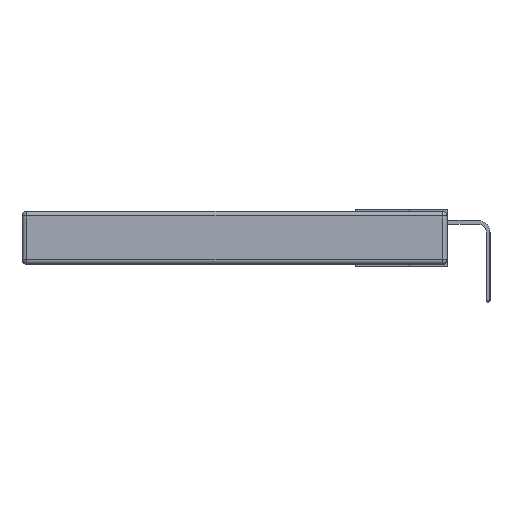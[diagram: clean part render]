
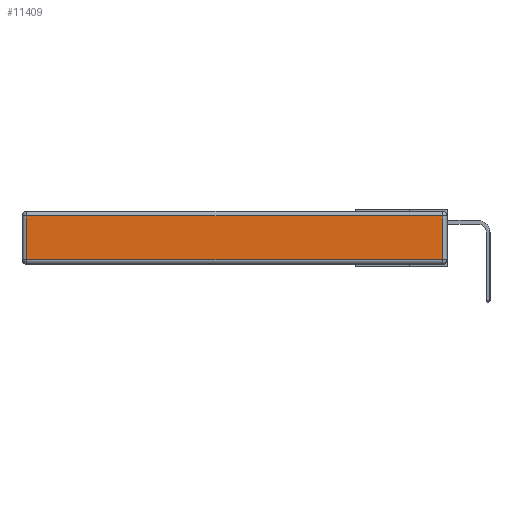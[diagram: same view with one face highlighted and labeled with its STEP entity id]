
A CAD part, left-side view. The second image highlights one B-rep face of the part: STEP entity #11409.
In plain terms, the highlighted planar face has unit normal (-1, 0, 0).
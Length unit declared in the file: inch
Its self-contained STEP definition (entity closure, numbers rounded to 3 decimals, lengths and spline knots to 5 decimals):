
#19 = DIRECTION ( 'NONE',  ( 0., 1., 0. ) ) ;
#1326 = LINE ( 'NONE', #7423, #20163 ) ;
#1357 = FACE_OUTER_BOUND ( 'NONE', #6916, .T. ) ;
#1763 = DIRECTION ( 'NONE',  ( 0., 0., -1. ) ) ;
#1868 = EDGE_CURVE ( 'NONE', #10426, #11444, #1326, .T. ) ;
#2377 = LINE ( 'NONE', #3318, #13028 ) ;
#3318 = CARTESIAN_POINT ( 'NONE',  ( 0., 2.75, -0.03 ) ) ;
#4161 = ORIENTED_EDGE ( 'NONE', *, *, #1868, .T. ) ;
#4529 = ORIENTED_EDGE ( 'NONE', *, *, #20145, .T. ) ;
#5215 = CARTESIAN_POINT ( 'NONE',  ( 0., 2.72, -0.343 ) ) ;
#5555 = PLANE ( 'NONE',  #19708 ) ;
#6508 = VERTEX_POINT ( 'NONE', #16748 ) ;
#6916 = EDGE_LOOP ( 'NONE', ( #4161, #12219, #12365, #4529 ) ) ;
#7284 = DIRECTION ( 'NONE',  ( -1., 0., 0. ) ) ;
#7423 = CARTESIAN_POINT ( 'NONE',  ( 0., 0., -0.313 ) ) ;
#7799 = LINE ( 'NONE', #5215, #8085 ) ;
#8085 = VECTOR ( 'NONE', #1763, 39.37008 ) ;
#8158 = CARTESIAN_POINT ( 'NONE',  ( 0., 0.03, -0.343 ) ) ;
#8367 = DIRECTION ( 'NONE',  ( 0., 0., 1. ) ) ;
#8727 = CARTESIAN_POINT ( 'NONE',  ( 0., 2.72, -0.03 ) ) ;
#10426 = VERTEX_POINT ( 'NONE', #17046 ) ;
#10549 = EDGE_CURVE ( 'NONE', #6508, #18899, #2377, .T. ) ;
#10748 = DIRECTION ( 'NONE',  ( 0., -1., 0. ) ) ;
#11409 = ADVANCED_FACE ( 'NONE', ( #1357 ), #5555, .T. ) ;
#11444 = VERTEX_POINT ( 'NONE', #19930 ) ;
#12219 = ORIENTED_EDGE ( 'NONE', *, *, #18809, .T. ) ;
#12365 = ORIENTED_EDGE ( 'NONE', *, *, #10549, .T. ) ;
#13028 = VECTOR ( 'NONE', #19, 39.37008 ) ;
#13633 = CARTESIAN_POINT ( 'NONE',  ( 0., 0., -0.343 ) ) ;
#16530 = DIRECTION ( 'NONE',  ( 0., 0., 1. ) ) ;
#16568 = LINE ( 'NONE', #8158, #19801 ) ;
#16748 = CARTESIAN_POINT ( 'NONE',  ( 0., 0.03, -0.03 ) ) ;
#17046 = CARTESIAN_POINT ( 'NONE',  ( 0., 2.72, -0.313 ) ) ;
#18809 = EDGE_CURVE ( 'NONE', #11444, #6508, #16568, .T. ) ;
#18899 = VERTEX_POINT ( 'NONE', #8727 ) ;
#19708 = AXIS2_PLACEMENT_3D ( 'NONE', #13633, #7284, #16530 ) ;
#19801 = VECTOR ( 'NONE', #8367, 39.37008 ) ;
#19930 = CARTESIAN_POINT ( 'NONE',  ( 0., 0.03, -0.313 ) ) ;
#20145 = EDGE_CURVE ( 'NONE', #18899, #10426, #7799, .T. ) ;
#20163 = VECTOR ( 'NONE', #10748, 39.37008 ) ;
